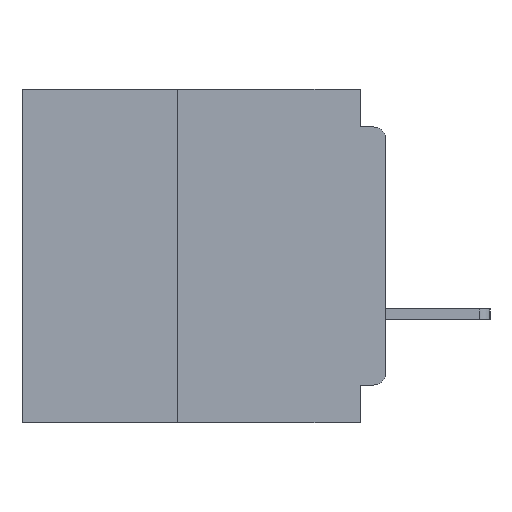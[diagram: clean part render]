
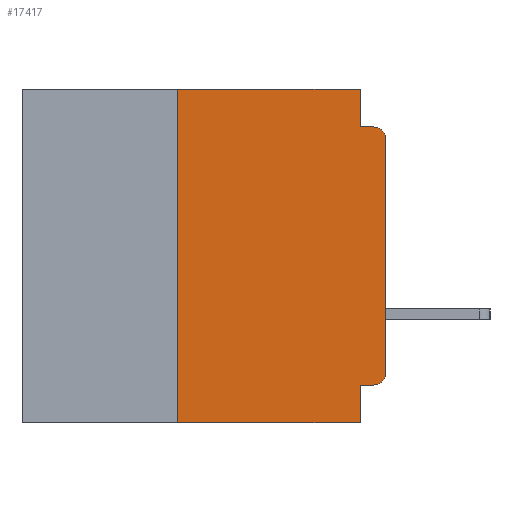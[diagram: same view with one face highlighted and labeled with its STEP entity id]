
A CAD part, left-side view. The second image highlights one B-rep face of the part: STEP entity #17417.
In plain terms, the highlighted planar face has unit normal (-1, 0, 0).
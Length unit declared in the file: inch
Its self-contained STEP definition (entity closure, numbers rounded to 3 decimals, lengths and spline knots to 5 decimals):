
#23 = EDGE_LOOP ( 'NONE', ( #27699, #20736, #1753, #21763, #11063, #32405, #19221, #20701, #13862, #755 ) ) ;
#755 = ORIENTED_EDGE ( 'NONE', *, *, #21022, .T. ) ;
#882 = CARTESIAN_POINT ( 'NONE',  ( 0., 0.437, 0. ) ) ;
#1615 = CARTESIAN_POINT ( 'NONE',  ( 0., 0.031, 0. ) ) ;
#1753 = ORIENTED_EDGE ( 'NONE', *, *, #13961, .F. ) ;
#2215 = EDGE_CURVE ( 'NONE', #25081, #35852, #30541, .T. ) ;
#2462 = VECTOR ( 'NONE', #37892, 39.37008 ) ;
#2771 = VERTEX_POINT ( 'NONE', #19066 ) ;
#3073 = DIRECTION ( 'NONE',  ( 0., 0., 1. ) ) ;
#4441 = LINE ( 'NONE', #10083, #2462 ) ;
#4923 = DIRECTION ( 'NONE',  ( 0., -1., 0. ) ) ;
#5849 = CARTESIAN_POINT ( 'NONE',  ( 0., 0.015, -0.355 ) ) ;
#5877 = VECTOR ( 'NONE', #4923, 39.37008 ) ;
#6412 = CARTESIAN_POINT ( 'NONE',  ( 0., 0., -0.06 ) ) ;
#7098 = CARTESIAN_POINT ( 'NONE',  ( 0., 0.031, -0.4 ) ) ;
#7457 = VECTOR ( 'NONE', #11637, 39.37008 ) ;
#7817 = FACE_OUTER_BOUND ( 'NONE', #23, .T. ) ;
#8085 = CARTESIAN_POINT ( 'NONE',  ( 0., 0.437, 0. ) ) ;
#8533 = CARTESIAN_POINT ( 'NONE',  ( 0., 0.25, -0.4 ) ) ;
#8769 = VECTOR ( 'NONE', #13350, 39.37008 ) ;
#8968 = AXIS2_PLACEMENT_3D ( 'NONE', #8085, #14354, #35900 ) ;
#9003 = CARTESIAN_POINT ( 'NONE',  ( 0., 0.031, 0. ) ) ;
#9512 = DIRECTION ( 'NONE',  ( -1., 0., 0. ) ) ;
#9733 = CARTESIAN_POINT ( 'NONE',  ( 0., 0., -0.34 ) ) ;
#10083 = CARTESIAN_POINT ( 'NONE',  ( 0., 0., -0.355 ) ) ;
#10409 = CARTESIAN_POINT ( 'NONE',  ( 0., 0.25, -0.4 ) ) ;
#11063 = ORIENTED_EDGE ( 'NONE', *, *, #2215, .F. ) ;
#11152 = CARTESIAN_POINT ( 'NONE',  ( 0., 0.25, 0. ) ) ;
#11637 = DIRECTION ( 'NONE',  ( 0., 0., 1. ) ) ;
#12030 = CARTESIAN_POINT ( 'NONE',  ( 0., 0., -0.045 ) ) ;
#12755 = AXIS2_PLACEMENT_3D ( 'NONE', #13760, #35342, #16921 ) ;
#12977 = VECTOR ( 'NONE', #23985, 39.37008 ) ;
#12979 = VERTEX_POINT ( 'NONE', #6412 ) ;
#13350 = DIRECTION ( 'NONE',  ( 0., 0., -1. ) ) ;
#13760 = CARTESIAN_POINT ( 'NONE',  ( 0., 0.015, -0.06 ) ) ;
#13862 = ORIENTED_EDGE ( 'NONE', *, *, #39501, .F. ) ;
#13961 = EDGE_CURVE ( 'NONE', #38091, #2771, #23142, .T. ) ;
#14354 = DIRECTION ( 'NONE',  ( 1., 0., 0. ) ) ;
#14908 = VECTOR ( 'NONE', #36736, 39.37008 ) ;
#15368 = VERTEX_POINT ( 'NONE', #9733 ) ;
#16483 = VERTEX_POINT ( 'NONE', #5849 ) ;
#16921 = DIRECTION ( 'NONE',  ( 0., 0., -1. ) ) ;
#17417 = ADVANCED_FACE ( 'NONE', ( #7817 ), #26638, .F. ) ;
#17863 = EDGE_CURVE ( 'NONE', #26985, #37927, #33433, .T. ) ;
#19066 = CARTESIAN_POINT ( 'NONE',  ( 0., 0.015, -0.045 ) ) ;
#19221 = ORIENTED_EDGE ( 'NONE', *, *, #22002, .T. ) ;
#19638 = CARTESIAN_POINT ( 'NONE',  ( 0., 0.031, -0.4 ) ) ;
#20701 = ORIENTED_EDGE ( 'NONE', *, *, #17863, .F. ) ;
#20736 = ORIENTED_EDGE ( 'NONE', *, *, #33355, .T. ) ;
#20915 = CARTESIAN_POINT ( 'NONE',  ( 0., 0.437, -0.4 ) ) ;
#21022 = EDGE_CURVE ( 'NONE', #16483, #15368, #28483, .T. ) ;
#21763 = ORIENTED_EDGE ( 'NONE', *, *, #28143, .F. ) ;
#22002 = EDGE_CURVE ( 'NONE', #23492, #37927, #37580, .T. ) ;
#23142 = LINE ( 'NONE', #12030, #14908 ) ;
#23444 = VECTOR ( 'NONE', #3073, 39.37008 ) ;
#23492 = VERTEX_POINT ( 'NONE', #10409 ) ;
#23985 = DIRECTION ( 'NONE',  ( 0., -1., 0. ) ) ;
#24070 = EDGE_CURVE ( 'NONE', #23492, #25081, #24917, .T. ) ;
#24917 = LINE ( 'NONE', #8533, #7457 ) ;
#25081 = VERTEX_POINT ( 'NONE', #11152 ) ;
#26638 = PLANE ( 'NONE',  #8968 ) ;
#26689 = AXIS2_PLACEMENT_3D ( 'NONE', #28052, #9512, #31131 ) ;
#26944 = VECTOR ( 'NONE', #29521, 39.37008 ) ;
#26985 = VERTEX_POINT ( 'NONE', #32976 ) ;
#27699 = ORIENTED_EDGE ( 'NONE', *, *, #38738, .T. ) ;
#28052 = CARTESIAN_POINT ( 'NONE',  ( 0., 0.015, -0.34 ) ) ;
#28143 = EDGE_CURVE ( 'NONE', #35852, #38091, #35126, .T. ) ;
#28483 = CIRCLE ( 'NONE', #26689, 0.015 ) ;
#29521 = DIRECTION ( 'NONE',  ( 0., 0., -1. ) ) ;
#30541 = LINE ( 'NONE', #882, #5877 ) ;
#31131 = DIRECTION ( 'NONE',  ( 0., 0., -1. ) ) ;
#31455 = CIRCLE ( 'NONE', #12755, 0.015 ) ;
#32405 = ORIENTED_EDGE ( 'NONE', *, *, #24070, .F. ) ;
#32558 = LINE ( 'NONE', #40053, #23444 ) ;
#32976 = CARTESIAN_POINT ( 'NONE',  ( 0., 0.031, -0.355 ) ) ;
#33355 = EDGE_CURVE ( 'NONE', #12979, #2771, #31455, .T. ) ;
#33433 = LINE ( 'NONE', #7098, #8769 ) ;
#35126 = LINE ( 'NONE', #1615, #26944 ) ;
#35342 = DIRECTION ( 'NONE',  ( -1., 0., 0. ) ) ;
#35852 = VERTEX_POINT ( 'NONE', #9003 ) ;
#35900 = DIRECTION ( 'NONE',  ( 0., 0., -1. ) ) ;
#36650 = CARTESIAN_POINT ( 'NONE',  ( 0., 0.031, -0.045 ) ) ;
#36736 = DIRECTION ( 'NONE',  ( 0., -1., 0. ) ) ;
#37580 = LINE ( 'NONE', #20915, #12977 ) ;
#37892 = DIRECTION ( 'NONE',  ( 0., 1., 0. ) ) ;
#37927 = VERTEX_POINT ( 'NONE', #19638 ) ;
#38091 = VERTEX_POINT ( 'NONE', #36650 ) ;
#38738 = EDGE_CURVE ( 'NONE', #15368, #12979, #32558, .T. ) ;
#39501 = EDGE_CURVE ( 'NONE', #16483, #26985, #4441, .T. ) ;
#40053 = CARTESIAN_POINT ( 'NONE',  ( 0., 0., 0. ) ) ;
